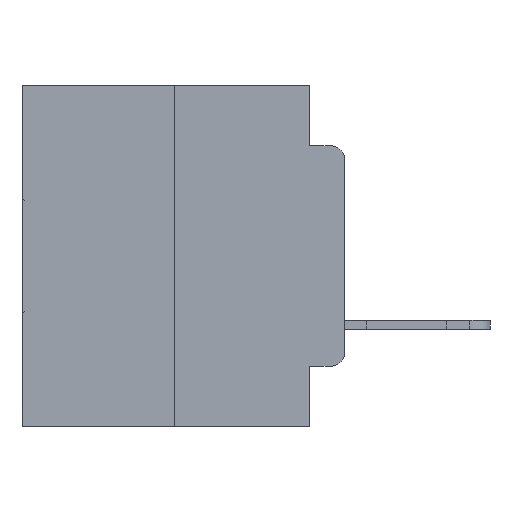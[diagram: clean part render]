
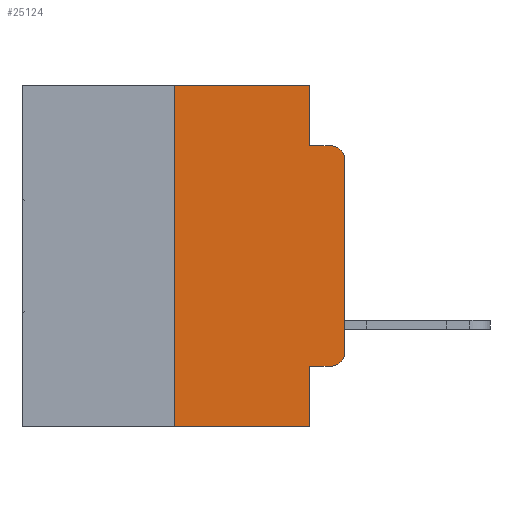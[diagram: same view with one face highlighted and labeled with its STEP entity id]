
A CAD part, left-side view. The second image highlights one B-rep face of the part: STEP entity #25124.
In plain terms, the highlighted planar face has unit normal (-1, 0, 0).
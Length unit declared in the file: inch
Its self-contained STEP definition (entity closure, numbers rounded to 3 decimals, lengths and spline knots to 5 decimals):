
#382 = VECTOR ( 'NONE', #10121, 39.37008 ) ;
#555 = ORIENTED_EDGE ( 'NONE', *, *, #3104, .F. ) ;
#606 = LINE ( 'NONE', #5620, #19965 ) ;
#692 = ORIENTED_EDGE ( 'NONE', *, *, #25101, .T. ) ;
#698 = DIRECTION ( 'NONE',  ( 1., 0., 0. ) ) ;
#1006 = ORIENTED_EDGE ( 'NONE', *, *, #8033, .F. ) ;
#1254 = AXIS2_PLACEMENT_3D ( 'NONE', #4253, #21022, #6720 ) ;
#1506 = ORIENTED_EDGE ( 'NONE', *, *, #9707, .T. ) ;
#1766 = CARTESIAN_POINT ( 'NONE',  ( 0., 0.051, -0.4115 ) ) ;
#2001 = ORIENTED_EDGE ( 'NONE', *, *, #14549, .T. ) ;
#2267 = VERTEX_POINT ( 'NONE', #3793 ) ;
#2491 = VECTOR ( 'NONE', #24525, 39.37008 ) ;
#2608 = VECTOR ( 'NONE', #22586, 39.37008 ) ;
#2617 = CARTESIAN_POINT ( 'NONE',  ( 0., 0.051, -0.5 ) ) ;
#3104 = EDGE_CURVE ( 'NONE', #13820, #13780, #25464, .T. ) ;
#3793 = CARTESIAN_POINT ( 'NONE',  ( 0., 0.02, -0.0885 ) ) ;
#4253 = CARTESIAN_POINT ( 'NONE',  ( 0., 0.02, -0.3915 ) ) ;
#4295 = EDGE_CURVE ( 'NONE', #13780, #22497, #6275, .T. ) ;
#4863 = CARTESIAN_POINT ( 'NONE',  ( 0., 0.25, 0. ) ) ;
#5620 = CARTESIAN_POINT ( 'NONE',  ( 0., 0.051, 0. ) ) ;
#5687 = VERTEX_POINT ( 'NONE', #28714 ) ;
#5967 = CARTESIAN_POINT ( 'NONE',  ( 0., 0., 0. ) ) ;
#6021 = ORIENTED_EDGE ( 'NONE', *, *, #16738, .T. ) ;
#6145 = DIRECTION ( 'NONE',  ( 0., -1., 0. ) ) ;
#6275 = LINE ( 'NONE', #9784, #28832 ) ;
#6720 = DIRECTION ( 'NONE',  ( 0., 0., -1. ) ) ;
#6902 = DIRECTION ( 'NONE',  ( 0., 0., 1. ) ) ;
#7587 = VERTEX_POINT ( 'NONE', #15708 ) ;
#8033 = EDGE_CURVE ( 'NONE', #16324, #10576, #12729, .T. ) ;
#8087 = CARTESIAN_POINT ( 'NONE',  ( 0., 0.473, 0. ) ) ;
#8385 = LINE ( 'NONE', #5967, #2608 ) ;
#8726 = VERTEX_POINT ( 'NONE', #26701 ) ;
#9059 = LINE ( 'NONE', #22311, #2491 ) ;
#9087 = CARTESIAN_POINT ( 'NONE',  ( 0., 0.051, -0.4115 ) ) ;
#9406 = AXIS2_PLACEMENT_3D ( 'NONE', #8087, #698, #17790 ) ;
#9707 = EDGE_CURVE ( 'NONE', #16324, #8726, #22910, .T. ) ;
#9784 = CARTESIAN_POINT ( 'NONE',  ( 0., 0.473, 0. ) ) ;
#10121 = DIRECTION ( 'NONE',  ( 0., 0., -1. ) ) ;
#10455 = CARTESIAN_POINT ( 'NONE',  ( 0., 0.051, 0. ) ) ;
#10576 = VERTEX_POINT ( 'NONE', #2617 ) ;
#11237 = DIRECTION ( 'NONE',  ( 0., -1., 0. ) ) ;
#12560 = CARTESIAN_POINT ( 'NONE',  ( 0., 0.25, 0. ) ) ;
#12729 = LINE ( 'NONE', #26359, #382 ) ;
#12847 = ORIENTED_EDGE ( 'NONE', *, *, #18338, .T. ) ;
#13262 = ORIENTED_EDGE ( 'NONE', *, *, #21405, .F. ) ;
#13780 = VERTEX_POINT ( 'NONE', #4863 ) ;
#13820 = VERTEX_POINT ( 'NONE', #26247 ) ;
#13948 = VECTOR ( 'NONE', #6902, 39.37008 ) ;
#13997 = DIRECTION ( 'NONE',  ( 0., -1., 0. ) ) ;
#14177 = CARTESIAN_POINT ( 'NONE',  ( 0., 0., -0.3915 ) ) ;
#14213 = DIRECTION ( 'NONE',  ( -1., 0., 0. ) ) ;
#14549 = EDGE_CURVE ( 'NONE', #8726, #18962, #24639, .T. ) ;
#15708 = CARTESIAN_POINT ( 'NONE',  ( 0., 0., -0.1085 ) ) ;
#16324 = VERTEX_POINT ( 'NONE', #9087 ) ;
#16738 = EDGE_CURVE ( 'NONE', #18962, #7587, #8385, .T. ) ;
#17387 = ORIENTED_EDGE ( 'NONE', *, *, #28814, .F. ) ;
#17790 = DIRECTION ( 'NONE',  ( 0., 0., -1. ) ) ;
#18338 = EDGE_CURVE ( 'NONE', #7587, #2267, #26524, .T. ) ;
#18962 = VERTEX_POINT ( 'NONE', #14177 ) ;
#19961 = DIRECTION ( 'NONE',  ( 0., 0., -1. ) ) ;
#19965 = VECTOR ( 'NONE', #19961, 39.37008 ) ;
#20945 = FACE_OUTER_BOUND ( 'NONE', #29313, .T. ) ;
#21008 = ORIENTED_EDGE ( 'NONE', *, *, #4295, .F. ) ;
#21022 = DIRECTION ( 'NONE',  ( -1., 0., 0. ) ) ;
#21405 = EDGE_CURVE ( 'NONE', #5687, #2267, #26651, .T. ) ;
#21447 = VECTOR ( 'NONE', #6145, 39.37008 ) ;
#22311 = CARTESIAN_POINT ( 'NONE',  ( 0., 0.473, -0.5 ) ) ;
#22497 = VERTEX_POINT ( 'NONE', #10455 ) ;
#22586 = DIRECTION ( 'NONE',  ( 0., 0., 1. ) ) ;
#22742 = CARTESIAN_POINT ( 'NONE',  ( 0., 0.051, -0.0885 ) ) ;
#22910 = LINE ( 'NONE', #1766, #24300 ) ;
#24300 = VECTOR ( 'NONE', #13997, 39.37008 ) ;
#24525 = DIRECTION ( 'NONE',  ( 0., -1., 0. ) ) ;
#24639 = CIRCLE ( 'NONE', #1254, 0.02 ) ;
#25101 = EDGE_CURVE ( 'NONE', #13820, #10576, #9059, .T. ) ;
#25124 = ADVANCED_FACE ( 'NONE', ( #20945 ), #28950, .F. ) ;
#25464 = LINE ( 'NONE', #12560, #13948 ) ;
#26247 = CARTESIAN_POINT ( 'NONE',  ( 0., 0.25, -0.5 ) ) ;
#26359 = CARTESIAN_POINT ( 'NONE',  ( 0., 0.051, 0. ) ) ;
#26419 = AXIS2_PLACEMENT_3D ( 'NONE', #27887, #14213, #30067 ) ;
#26524 = CIRCLE ( 'NONE', #26419, 0.02 ) ;
#26651 = LINE ( 'NONE', #22742, #21447 ) ;
#26701 = CARTESIAN_POINT ( 'NONE',  ( 0., 0.02, -0.4115 ) ) ;
#27887 = CARTESIAN_POINT ( 'NONE',  ( 0., 0.02, -0.1085 ) ) ;
#28714 = CARTESIAN_POINT ( 'NONE',  ( 0., 0.051, -0.0885 ) ) ;
#28814 = EDGE_CURVE ( 'NONE', #22497, #5687, #606, .T. ) ;
#28832 = VECTOR ( 'NONE', #11237, 39.37008 ) ;
#28950 = PLANE ( 'NONE',  #9406 ) ;
#29313 = EDGE_LOOP ( 'NONE', ( #6021, #12847, #13262, #17387, #21008, #555, #692, #1006, #1506, #2001 ) ) ;
#30067 = DIRECTION ( 'NONE',  ( 0., 0., -1. ) ) ;
